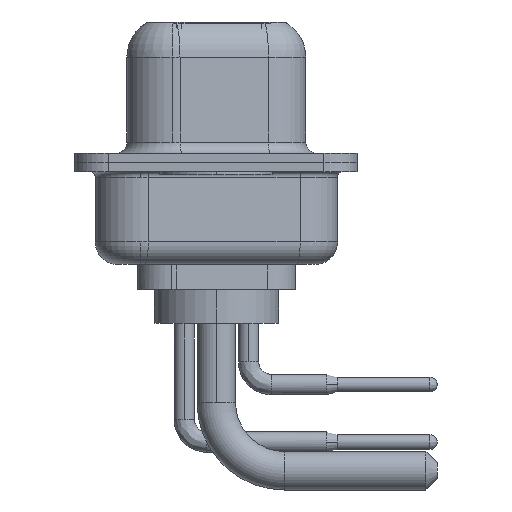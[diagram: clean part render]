
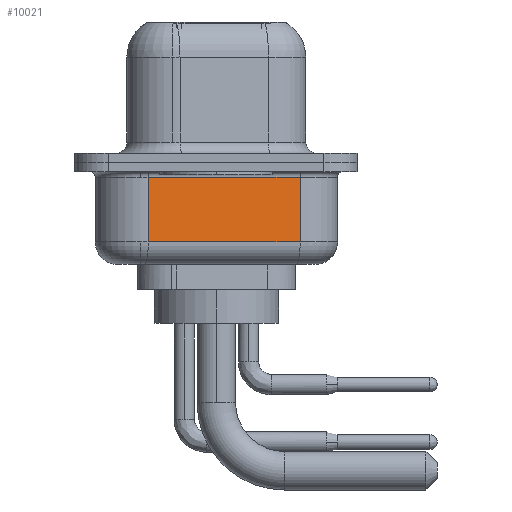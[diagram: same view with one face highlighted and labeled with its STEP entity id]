
A CAD part, left-side view. The second image highlights one B-rep face of the part: STEP entity #10021.
In plain terms, the highlighted planar face has unit normal (-0.985, -0.174, 0).
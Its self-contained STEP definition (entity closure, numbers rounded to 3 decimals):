
#555 = VERTEX_POINT ( 'NONE', #14560 ) ;
#778 = DIRECTION ( 'NONE',  ( 0.985, 0.174, 0. ) ) ;
#856 = DIRECTION ( 'NONE',  ( 0., 0., 1. ) ) ;
#976 = VECTOR ( 'NONE', #7141, 1000. ) ;
#1016 = VERTEX_POINT ( 'NONE', #15936 ) ;
#1107 = VECTOR ( 'NONE', #856, 1000. ) ;
#1217 = LINE ( 'NONE', #5603, #16980 ) ;
#1461 = LINE ( 'NONE', #14062, #976 ) ;
#1524 = AXIS2_PLACEMENT_3D ( 'NONE', #2541, #778, #12142 ) ;
#1977 = CARTESIAN_POINT ( 'NONE',  ( 4.062, -3.697, -4.5 ) ) ;
#2309 = DIRECTION ( 'NONE',  ( 0., 0., 1. ) ) ;
#2541 = CARTESIAN_POINT ( 'NONE',  ( 2.88, 3.003, -4.5 ) ) ;
#4015 = EDGE_CURVE ( 'NONE', #555, #9678, #14750, .T. ) ;
#4606 = ORIENTED_EDGE ( 'NONE', *, *, #11980, .T. ) ;
#5121 = CARTESIAN_POINT ( 'NONE',  ( 2.88, 3.003, -4.5 ) ) ;
#5603 = CARTESIAN_POINT ( 'NONE',  ( 2.88, 3.003, -3.5 ) ) ;
#6735 = PLANE ( 'NONE',  #1524 ) ;
#7141 = DIRECTION ( 'NONE',  ( -0.174, 0.985, 0. ) ) ;
#8138 = FACE_OUTER_BOUND ( 'NONE', #9384, .T. ) ;
#9330 = EDGE_CURVE ( 'NONE', #18336, #555, #1217, .T. ) ;
#9384 = EDGE_LOOP ( 'NONE', ( #18012, #9457, #15197, #4606 ) ) ;
#9457 = ORIENTED_EDGE ( 'NONE', *, *, #9330, .T. ) ;
#9678 = VERTEX_POINT ( 'NONE', #9749 ) ;
#9749 = CARTESIAN_POINT ( 'NONE',  ( 4.062, -3.697, -0.65 ) ) ;
#10021 = ADVANCED_FACE ( 'NONE', ( #8138 ), #6735, .F. ) ;
#11980 = EDGE_CURVE ( 'NONE', #9678, #1016, #1461, .T. ) ;
#12142 = DIRECTION ( 'NONE',  ( -0.174, 0.985, 0. ) ) ;
#14062 = CARTESIAN_POINT ( 'NONE',  ( 2.88, 3.003, -0.65 ) ) ;
#14560 = CARTESIAN_POINT ( 'NONE',  ( 4.062, -3.697, -3.5 ) ) ;
#14750 = LINE ( 'NONE', #1977, #1107 ) ;
#15197 = ORIENTED_EDGE ( 'NONE', *, *, #4015, .T. ) ;
#15936 = CARTESIAN_POINT ( 'NONE',  ( 2.88, 3.003, -0.65 ) ) ;
#16724 = CARTESIAN_POINT ( 'NONE',  ( 2.88, 3.003, -3.5 ) ) ;
#16791 = DIRECTION ( 'NONE',  ( 0.174, -0.985, 0. ) ) ;
#16980 = VECTOR ( 'NONE', #16791, 1000. ) ;
#17343 = EDGE_CURVE ( 'NONE', #18336, #1016, #17912, .T. ) ;
#17779 = VECTOR ( 'NONE', #2309, 1000. ) ;
#17912 = LINE ( 'NONE', #5121, #17779 ) ;
#18012 = ORIENTED_EDGE ( 'NONE', *, *, #17343, .F. ) ;
#18336 = VERTEX_POINT ( 'NONE', #16724 ) ;
